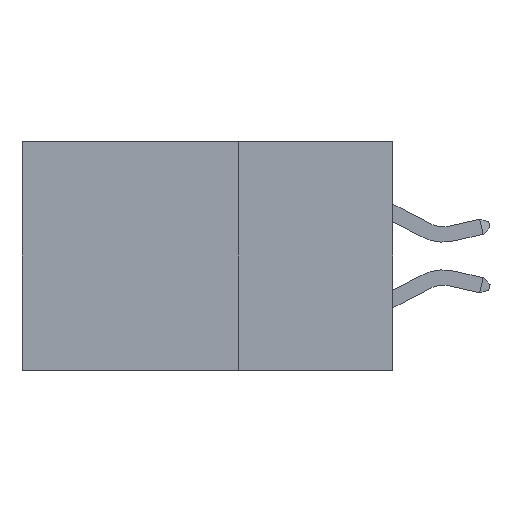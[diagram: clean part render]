
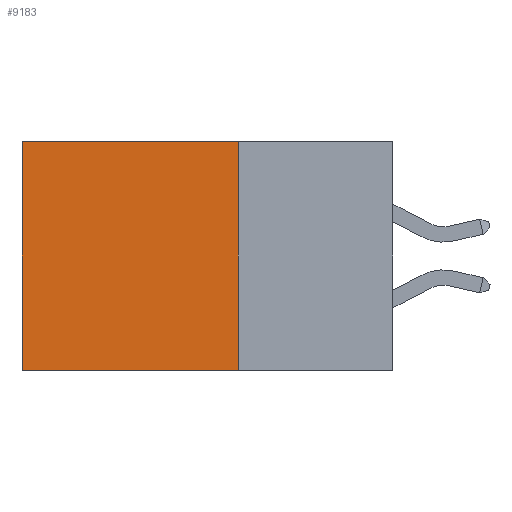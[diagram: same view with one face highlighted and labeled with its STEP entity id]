
A CAD part, left-side view. The second image highlights one B-rep face of the part: STEP entity #9183.
In plain terms, the highlighted planar face has unit normal (-1, 0, 0).
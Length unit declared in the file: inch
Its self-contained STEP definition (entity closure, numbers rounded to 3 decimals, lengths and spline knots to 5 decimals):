
#167 = VERTEX_POINT ( 'NONE', #17545 ) ;
#1359 = EDGE_CURVE ( 'NONE', #4249, #18532, #4759, .T. ) ;
#1606 = ORIENTED_EDGE ( 'NONE', *, *, #16406, .T. ) ;
#1634 = VECTOR ( 'NONE', #12851, 39.37008 ) ;
#1889 = AXIS2_PLACEMENT_3D ( 'NONE', #16837, #10694, #9107 ) ;
#2685 = CARTESIAN_POINT ( 'NONE',  ( 0.2875, 0.6, 0. ) ) ;
#2688 = LINE ( 'NONE', #2685, #14664 ) ;
#3939 = ORIENTED_EDGE ( 'NONE', *, *, #11467, .F. ) ;
#4052 = DIRECTION ( 'NONE',  ( 0., 1., 0. ) ) ;
#4072 = PLANE ( 'NONE',  #1889 ) ;
#4249 = VERTEX_POINT ( 'NONE', #4788 ) ;
#4678 = EDGE_LOOP ( 'NONE', ( #1606, #3939, #19740, #9575 ) ) ;
#4759 = LINE ( 'NONE', #6667, #1634 ) ;
#4788 = CARTESIAN_POINT ( 'NONE',  ( 0.2875, 0.25, 0. ) ) ;
#6667 = CARTESIAN_POINT ( 'NONE',  ( 0.2875, 0.25, 0. ) ) ;
#6668 = CARTESIAN_POINT ( 'NONE',  ( 0.2875, 0.25, 0. ) ) ;
#8419 = VECTOR ( 'NONE', #12480, 39.37008 ) ;
#8564 = FACE_OUTER_BOUND ( 'NONE', #4678, .T. ) ;
#9107 = DIRECTION ( 'NONE',  ( 0., 0., -1. ) ) ;
#9183 = ADVANCED_FACE ( 'NONE', ( #8564 ), #4072, .F. ) ;
#9575 = ORIENTED_EDGE ( 'NONE', *, *, #12836, .T. ) ;
#10694 = DIRECTION ( 'NONE',  ( 1., 0., 0. ) ) ;
#10848 = VERTEX_POINT ( 'NONE', #18298 ) ;
#11467 = EDGE_CURVE ( 'NONE', #18532, #167, #19859, .T. ) ;
#12093 = DIRECTION ( 'NONE',  ( 0., 0., -1. ) ) ;
#12260 = LINE ( 'NONE', #6668, #20061 ) ;
#12413 = CARTESIAN_POINT ( 'NONE',  ( 0.2875, 0.25, -0.37 ) ) ;
#12480 = DIRECTION ( 'NONE',  ( 0., 1., 0. ) ) ;
#12836 = EDGE_CURVE ( 'NONE', #4249, #10848, #12260, .T. ) ;
#12851 = DIRECTION ( 'NONE',  ( 0., 0., -1. ) ) ;
#14664 = VECTOR ( 'NONE', #12093, 39.37008 ) ;
#16406 = EDGE_CURVE ( 'NONE', #10848, #167, #2688, .T. ) ;
#16837 = CARTESIAN_POINT ( 'NONE',  ( 0.2875, 0.25, 0. ) ) ;
#17545 = CARTESIAN_POINT ( 'NONE',  ( 0.2875, 0.6, -0.37 ) ) ;
#18298 = CARTESIAN_POINT ( 'NONE',  ( 0.2875, 0.6, 0. ) ) ;
#18532 = VERTEX_POINT ( 'NONE', #19393 ) ;
#19393 = CARTESIAN_POINT ( 'NONE',  ( 0.2875, 0.25, -0.37 ) ) ;
#19740 = ORIENTED_EDGE ( 'NONE', *, *, #1359, .F. ) ;
#19859 = LINE ( 'NONE', #12413, #8419 ) ;
#20061 = VECTOR ( 'NONE', #4052, 39.37008 ) ;
